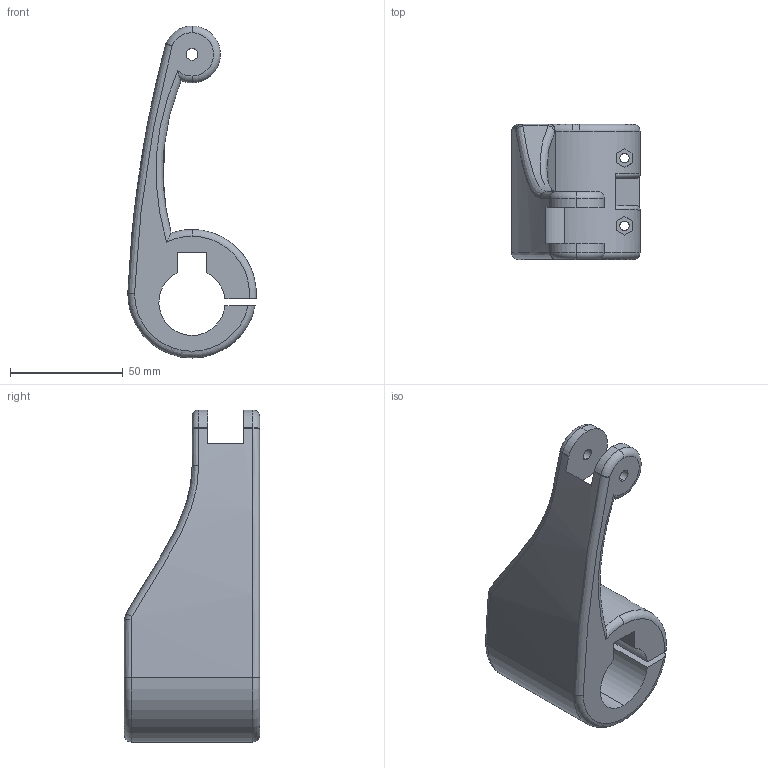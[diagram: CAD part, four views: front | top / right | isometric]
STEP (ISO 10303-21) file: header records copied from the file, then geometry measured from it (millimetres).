
FILE_DESCRIPTION (( 'STEP AP203' ), '1' );
FILE_NAME ('BodyL.STEP', '2020-10-24T03:16:12', ( '' ), ( '' ), 'SwSTEP 2.0', 'SolidWorks 2019', '' );
FILE_SCHEMA (( 'CONFIG_CONTROL_DESIGN' ));
Length unit declared in the file: millimetre
Products named in the file (1): BodyL
Bounding box: 57 x 60 x 147.3 mm (x, y, z)
Volume: 144538.8 mm3; surface area: 33042.1 mm2
Topology: 1 solids, 1 shells, 105 faces, 267 edges, 169 vertices
Faces by surface type: cylinder 37, plane 37, torus 15, bspline 14, sphere 2
Entity records: 4151 total; most frequent: CARTESIAN_POINT 1596, ORIENTED_EDGE 532, DIRECTION 499, EDGE_CURVE 266, AXIS2_PLACEMENT_3D 194, VERTEX_POINT 169, EDGE_LOOP 123, VECTOR 111
